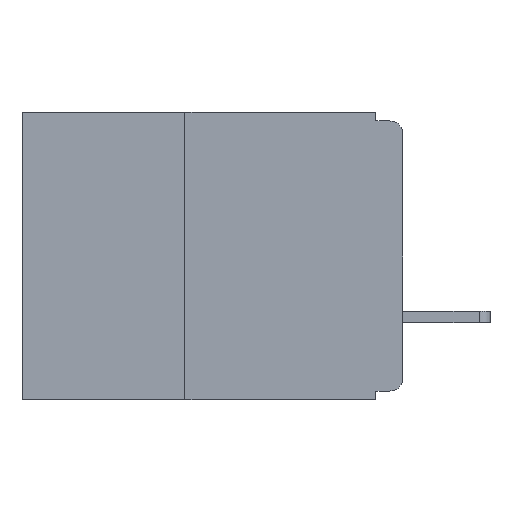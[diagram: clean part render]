
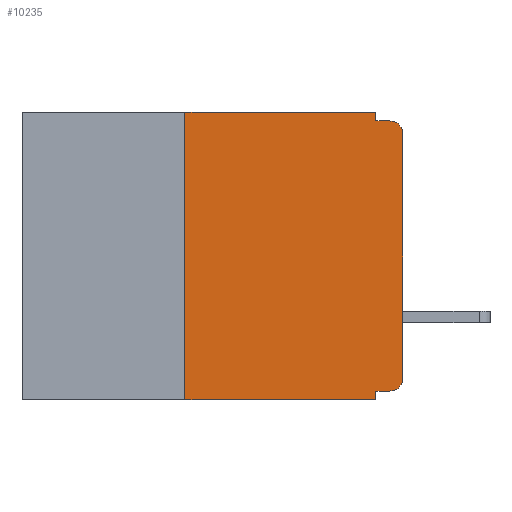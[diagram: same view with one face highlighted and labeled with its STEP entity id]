
A CAD part, left-side view. The second image highlights one B-rep face of the part: STEP entity #10235.
In plain terms, the highlighted planar face has unit normal (-1, 0, 0).
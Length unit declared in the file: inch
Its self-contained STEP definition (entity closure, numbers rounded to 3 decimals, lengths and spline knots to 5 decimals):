
#26 = ORIENTED_EDGE ( 'NONE', *, *, #3606, .T. ) ;
#31 = VECTOR ( 'NONE', #27436, 39.37008 ) ;
#142 = LINE ( 'NONE', #27428, #6997 ) ;
#304 = VECTOR ( 'NONE', #27657, 39.37008 ) ;
#411 = ORIENTED_EDGE ( 'NONE', *, *, #12756, .F. ) ;
#1218 = EDGE_CURVE ( 'NONE', #23586, #17820, #10008, .T. ) ;
#1306 = CARTESIAN_POINT ( 'NONE',  ( 0., 0.015, -0.01 ) ) ;
#1625 = CARTESIAN_POINT ( 'NONE',  ( 0., 0., -0.025 ) ) ;
#2777 = VERTEX_POINT ( 'NONE', #27702 ) ;
#3289 = VECTOR ( 'NONE', #12748, 39.37008 ) ;
#3606 = EDGE_CURVE ( 'NONE', #22442, #17110, #27110, .T. ) ;
#3649 = AXIS2_PLACEMENT_3D ( 'NONE', #10797, #28566, #13378 ) ;
#3807 = ORIENTED_EDGE ( 'NONE', *, *, #1218, .T. ) ;
#4353 = DIRECTION ( 'NONE',  ( 0., 0., -1. ) ) ;
#4648 = VERTEX_POINT ( 'NONE', #31542 ) ;
#4684 = ORIENTED_EDGE ( 'NONE', *, *, #21316, .F. ) ;
#5060 = ORIENTED_EDGE ( 'NONE', *, *, #19272, .F. ) ;
#6341 = DIRECTION ( 'NONE',  ( 1., 0., 0. ) ) ;
#6997 = VECTOR ( 'NONE', #24886, 39.37008 ) ;
#7102 = DIRECTION ( 'NONE',  ( 0., -1., 0. ) ) ;
#7278 = CARTESIAN_POINT ( 'NONE',  ( 0., 0.25, -0.33 ) ) ;
#7958 = LINE ( 'NONE', #20049, #304 ) ;
#8690 = LINE ( 'NONE', #19591, #22204 ) ;
#9588 = ORIENTED_EDGE ( 'NONE', *, *, #27531, .F. ) ;
#10008 = LINE ( 'NONE', #12603, #3289 ) ;
#10235 = ADVANCED_FACE ( 'NONE', ( #12760 ), #21575, .F. ) ;
#10308 = CARTESIAN_POINT ( 'NONE',  ( 0., 0.437, 0. ) ) ;
#10797 = CARTESIAN_POINT ( 'NONE',  ( 0., 0.015, -0.305 ) ) ;
#11807 = AXIS2_PLACEMENT_3D ( 'NONE', #28634, #13442, #31151 ) ;
#11885 = EDGE_CURVE ( 'NONE', #17820, #13976, #23844, .T. ) ;
#12132 = DIRECTION ( 'NONE',  ( 0., 0., -1. ) ) ;
#12248 = ORIENTED_EDGE ( 'NONE', *, *, #11885, .T. ) ;
#12378 = VERTEX_POINT ( 'NONE', #27993 ) ;
#12603 = CARTESIAN_POINT ( 'NONE',  ( 0., 0., 0. ) ) ;
#12748 = DIRECTION ( 'NONE',  ( 0., 0., 1. ) ) ;
#12756 = EDGE_CURVE ( 'NONE', #32394, #17110, #8690, .T. ) ;
#12760 = FACE_OUTER_BOUND ( 'NONE', #15886, .T. ) ;
#12881 = DIRECTION ( 'NONE',  ( 0., -1., 0. ) ) ;
#13378 = DIRECTION ( 'NONE',  ( 0., 0., -1. ) ) ;
#13385 = VECTOR ( 'NONE', #12132, 39.37008 ) ;
#13442 = DIRECTION ( 'NONE',  ( -1., 0., 0. ) ) ;
#13484 = EDGE_CURVE ( 'NONE', #24865, #12378, #26863, .T. ) ;
#13976 = VERTEX_POINT ( 'NONE', #1306 ) ;
#14169 = EDGE_CURVE ( 'NONE', #22442, #4648, #142, .T. ) ;
#15886 = EDGE_LOOP ( 'NONE', ( #3807, #12248, #9588, #31344, #4684, #18750, #26, #411, #5060, #30806 ) ) ;
#16461 = CARTESIAN_POINT ( 'NONE',  ( 0., 0.437, 0. ) ) ;
#17110 = VERTEX_POINT ( 'NONE', #19482 ) ;
#17287 = CARTESIAN_POINT ( 'NONE',  ( 0., 0., -0.305 ) ) ;
#17820 = VERTEX_POINT ( 'NONE', #1625 ) ;
#18073 = LINE ( 'NONE', #10308, #23234 ) ;
#18750 = ORIENTED_EDGE ( 'NONE', *, *, #14169, .F. ) ;
#18875 = EDGE_CURVE ( 'NONE', #2777, #23586, #25834, .T. ) ;
#19272 = EDGE_CURVE ( 'NONE', #2777, #32394, #7958, .T. ) ;
#19482 = CARTESIAN_POINT ( 'NONE',  ( 0., 0.031, -0.33 ) ) ;
#19591 = CARTESIAN_POINT ( 'NONE',  ( 0., 0.031, -0.33 ) ) ;
#19781 = CARTESIAN_POINT ( 'NONE',  ( 0., 0., -0.01 ) ) ;
#20049 = CARTESIAN_POINT ( 'NONE',  ( 0., 0., -0.32 ) ) ;
#21230 = LINE ( 'NONE', #19781, #27120 ) ;
#21316 = EDGE_CURVE ( 'NONE', #4648, #24865, #18073, .T. ) ;
#21575 = PLANE ( 'NONE',  #22461 ) ;
#22204 = VECTOR ( 'NONE', #4353, 39.37008 ) ;
#22442 = VERTEX_POINT ( 'NONE', #7278 ) ;
#22461 = AXIS2_PLACEMENT_3D ( 'NONE', #16461, #6341, #24095 ) ;
#23234 = VECTOR ( 'NONE', #12881, 39.37008 ) ;
#23586 = VERTEX_POINT ( 'NONE', #17287 ) ;
#23844 = CIRCLE ( 'NONE', #11807, 0.015 ) ;
#24095 = DIRECTION ( 'NONE',  ( 0., 0., -1. ) ) ;
#24865 = VERTEX_POINT ( 'NONE', #25410 ) ;
#24886 = DIRECTION ( 'NONE',  ( 0., 0., 1. ) ) ;
#24891 = CARTESIAN_POINT ( 'NONE',  ( 0., 0.437, -0.33 ) ) ;
#25410 = CARTESIAN_POINT ( 'NONE',  ( 0., 0.031, 0. ) ) ;
#25834 = CIRCLE ( 'NONE', #3649, 0.015 ) ;
#26863 = LINE ( 'NONE', #32276, #13385 ) ;
#27110 = LINE ( 'NONE', #24891, #31 ) ;
#27120 = VECTOR ( 'NONE', #7102, 39.37008 ) ;
#27428 = CARTESIAN_POINT ( 'NONE',  ( 0., 0.25, -0.33 ) ) ;
#27436 = DIRECTION ( 'NONE',  ( 0., -1., 0. ) ) ;
#27531 = EDGE_CURVE ( 'NONE', #12378, #13976, #21230, .T. ) ;
#27657 = DIRECTION ( 'NONE',  ( 0., 1., 0. ) ) ;
#27702 = CARTESIAN_POINT ( 'NONE',  ( 0., 0.015, -0.32 ) ) ;
#27992 = CARTESIAN_POINT ( 'NONE',  ( 0., 0.031, -0.32 ) ) ;
#27993 = CARTESIAN_POINT ( 'NONE',  ( 0., 0.031, -0.01 ) ) ;
#28566 = DIRECTION ( 'NONE',  ( -1., 0., 0. ) ) ;
#28634 = CARTESIAN_POINT ( 'NONE',  ( 0., 0.015, -0.025 ) ) ;
#30806 = ORIENTED_EDGE ( 'NONE', *, *, #18875, .T. ) ;
#31151 = DIRECTION ( 'NONE',  ( 0., 0., -1. ) ) ;
#31344 = ORIENTED_EDGE ( 'NONE', *, *, #13484, .F. ) ;
#31542 = CARTESIAN_POINT ( 'NONE',  ( 0., 0.25, 0. ) ) ;
#32276 = CARTESIAN_POINT ( 'NONE',  ( 0., 0.031, 0. ) ) ;
#32394 = VERTEX_POINT ( 'NONE', #27992 ) ;
